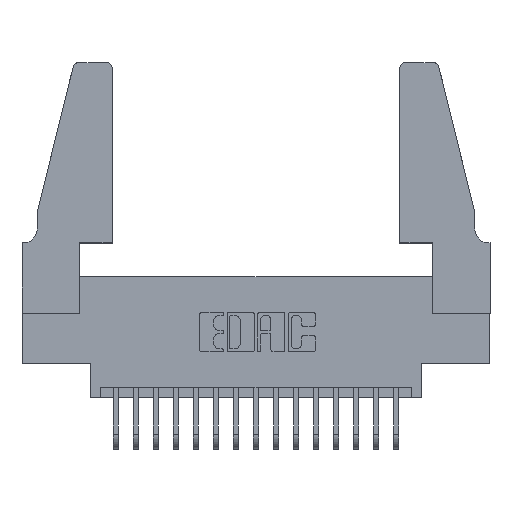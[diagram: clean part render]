
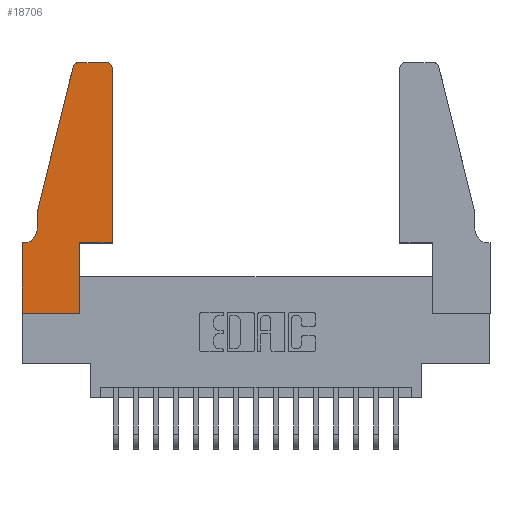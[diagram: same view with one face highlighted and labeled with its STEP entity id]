
A CAD part, top view. The second image highlights one B-rep face of the part: STEP entity #18706.
In plain terms, the highlighted planar face has unit normal (0, 0, 1).
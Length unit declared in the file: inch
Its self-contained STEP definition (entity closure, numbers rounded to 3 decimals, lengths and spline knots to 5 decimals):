
#60 = DIRECTION ( 'NONE',  ( -0.239, -0.971, 0. ) ) ;
#128 = CARTESIAN_POINT ( 'NONE',  ( 0.4505, 0.35, 0.37 ) ) ;
#160 = EDGE_CURVE ( 'NONE', #6069, #14616, #15178, .T. ) ;
#247 = EDGE_CURVE ( 'NONE', #14616, #1407, #3761, .T. ) ;
#434 = CIRCLE ( 'NONE', #5238, 0.03 ) ;
#468 = VECTOR ( 'NONE', #3571, 39.37008 ) ;
#499 = CARTESIAN_POINT ( 'NONE',  ( 0.0055, 0.42, 0.37 ) ) ;
#738 = CIRCLE ( 'NONE', #7041, 0.07 ) ;
#1019 = DIRECTION ( 'NONE',  ( 0., 0., 1. ) ) ;
#1141 = DIRECTION ( 'NONE',  ( -1., 0., 0. ) ) ;
#1270 = VERTEX_POINT ( 'NONE', #17193 ) ;
#1292 = VECTOR ( 'NONE', #11896, 39.37008 ) ;
#1400 = FACE_OUTER_BOUND ( 'NONE', #6857, .T. ) ;
#1407 = VERTEX_POINT ( 'NONE', #5744 ) ;
#1433 = CARTESIAN_POINT ( 'NONE',  ( 0.4505, 0.35, 0.37 ) ) ;
#1527 = EDGE_CURVE ( 'NONE', #12552, #3239, #3700, .T. ) ;
#1777 = VECTOR ( 'NONE', #12520, 39.37008 ) ;
#1873 = VECTOR ( 'NONE', #1141, 39.37008 ) ;
#2265 = VERTEX_POINT ( 'NONE', #14959 ) ;
#2568 = PLANE ( 'NONE',  #15104 ) ;
#2570 = VERTEX_POINT ( 'NONE', #6822 ) ;
#2880 = ORIENTED_EDGE ( 'NONE', *, *, #13255, .T. ) ;
#3009 = ORIENTED_EDGE ( 'NONE', *, *, #9297, .T. ) ;
#3200 = DIRECTION ( 'NONE',  ( 0., -1., 0. ) ) ;
#3239 = VERTEX_POINT ( 'NONE', #16061 ) ;
#3508 = CARTESIAN_POINT ( 'NONE',  ( 0.0755, 0.35, 0.37 ) ) ;
#3571 = DIRECTION ( 'NONE',  ( 1., 0., 0. ) ) ;
#3700 = LINE ( 'NONE', #17986, #8347 ) ;
#3761 = LINE ( 'NONE', #16652, #14265 ) ;
#3788 = ORIENTED_EDGE ( 'NONE', *, *, #7054, .T. ) ;
#4118 = DIRECTION ( 'NONE',  ( 0., 0., 1. ) ) ;
#4367 = LINE ( 'NONE', #3508, #1777 ) ;
#5176 = VECTOR ( 'NONE', #14884, 39.37008 ) ;
#5238 = AXIS2_PLACEMENT_3D ( 'NONE', #15968, #1019, #5418 ) ;
#5287 = LINE ( 'NONE', #1433, #1292 ) ;
#5418 = DIRECTION ( 'NONE',  ( 1., 0., 0. ) ) ;
#5697 = DIRECTION ( 'NONE',  ( 1., 0., 0. ) ) ;
#5744 = CARTESIAN_POINT ( 'NONE',  ( 0.2865, 0.35, 0.37 ) ) ;
#5806 = ORIENTED_EDGE ( 'NONE', *, *, #18556, .T. ) ;
#6069 = VERTEX_POINT ( 'NONE', #8183 ) ;
#6198 = ORIENTED_EDGE ( 'NONE', *, *, #1527, .T. ) ;
#6437 = ORIENTED_EDGE ( 'NONE', *, *, #14283, .T. ) ;
#6822 = CARTESIAN_POINT ( 'NONE',  ( 0.0755, 0.42, 0.37 ) ) ;
#6857 = EDGE_LOOP ( 'NONE', ( #16864, #3788, #6198, #16305, #12976, #6437, #3009, #13708, #15267, #5806, #18060, #2880 ) ) ;
#6881 = CARTESIAN_POINT ( 'NONE',  ( 0.25487, 1.22718, 0.37 ) ) ;
#7041 = AXIS2_PLACEMENT_3D ( 'NONE', #499, #16013, #14645 ) ;
#7054 = EDGE_CURVE ( 'NONE', #1270, #12552, #434, .T. ) ;
#7092 = DIRECTION ( 'NONE',  ( 0., 0., 1. ) ) ;
#7910 = VERTEX_POINT ( 'NONE', #15102 ) ;
#8183 = CARTESIAN_POINT ( 'NONE',  ( 0., 0., 0.37 ) ) ;
#8347 = VECTOR ( 'NONE', #60, 39.37008 ) ;
#8463 = EDGE_CURVE ( 'NONE', #3239, #2570, #17456, .T. ) ;
#8550 = LINE ( 'NONE', #18088, #10180 ) ;
#8596 = CARTESIAN_POINT ( 'NONE',  ( 0.0055, 0.35, 0.37 ) ) ;
#8775 = VERTEX_POINT ( 'NONE', #8596 ) ;
#9185 = EDGE_CURVE ( 'NONE', #17569, #19368, #5287, .T. ) ;
#9218 = DIRECTION ( 'NONE',  ( 0., 1., 0. ) ) ;
#9297 = EDGE_CURVE ( 'NONE', #7910, #6069, #8550, .T. ) ;
#10180 = VECTOR ( 'NONE', #3200, 39.37008 ) ;
#10377 = CARTESIAN_POINT ( 'NONE',  ( 0.4205, 1.22, 0.37 ) ) ;
#10914 = VECTOR ( 'NONE', #16899, 39.37008 ) ;
#10998 = EDGE_CURVE ( 'NONE', #2570, #8775, #738, .T. ) ;
#11688 = LINE ( 'NONE', #16017, #1873 ) ;
#11896 = DIRECTION ( 'NONE',  ( 0., 1., 0. ) ) ;
#12171 = LINE ( 'NONE', #14202, #468 ) ;
#12361 = EDGE_CURVE ( 'NONE', #2265, #1270, #11688, .T. ) ;
#12520 = DIRECTION ( 'NONE',  ( -1., 0., 0. ) ) ;
#12552 = VERTEX_POINT ( 'NONE', #6881 ) ;
#12976 = ORIENTED_EDGE ( 'NONE', *, *, #10998, .T. ) ;
#13255 = EDGE_CURVE ( 'NONE', #19368, #2265, #16784, .T. ) ;
#13708 = ORIENTED_EDGE ( 'NONE', *, *, #160, .T. ) ;
#14070 = AXIS2_PLACEMENT_3D ( 'NONE', #10377, #4118, #5697 ) ;
#14202 = CARTESIAN_POINT ( 'NONE',  ( 0.4505, 0.35, 0.37 ) ) ;
#14265 = VECTOR ( 'NONE', #9218, 39.37008 ) ;
#14268 = DIRECTION ( 'NONE',  ( 1., 0., 0. ) ) ;
#14283 = EDGE_CURVE ( 'NONE', #8775, #7910, #4367, .T. ) ;
#14616 = VERTEX_POINT ( 'NONE', #17322 ) ;
#14645 = DIRECTION ( 'NONE',  ( -1., 0., 0. ) ) ;
#14823 = CARTESIAN_POINT ( 'NONE',  ( 0., 0., 0.37 ) ) ;
#14884 = DIRECTION ( 'NONE',  ( 1., 0., 0. ) ) ;
#14959 = CARTESIAN_POINT ( 'NONE',  ( 0.4205, 1.25, 0.37 ) ) ;
#15102 = CARTESIAN_POINT ( 'NONE',  ( 0., 0.35, 0.37 ) ) ;
#15104 = AXIS2_PLACEMENT_3D ( 'NONE', #17271, #7092, #14268 ) ;
#15178 = LINE ( 'NONE', #14823, #5176 ) ;
#15267 = ORIENTED_EDGE ( 'NONE', *, *, #247, .T. ) ;
#15968 = CARTESIAN_POINT ( 'NONE',  ( 0.284, 1.22, 0.37 ) ) ;
#16013 = DIRECTION ( 'NONE',  ( 0., 0., -1. ) ) ;
#16017 = CARTESIAN_POINT ( 'NONE',  ( 0.2605, 1.25, 0.37 ) ) ;
#16061 = CARTESIAN_POINT ( 'NONE',  ( 0.0755, 0.5, 0.37 ) ) ;
#16305 = ORIENTED_EDGE ( 'NONE', *, *, #8463, .T. ) ;
#16652 = CARTESIAN_POINT ( 'NONE',  ( 0.2865, 0.35, 0.37 ) ) ;
#16784 = CIRCLE ( 'NONE', #14070, 0.03 ) ;
#16864 = ORIENTED_EDGE ( 'NONE', *, *, #12361, .T. ) ;
#16899 = DIRECTION ( 'NONE',  ( 0., -1., 0. ) ) ;
#17193 = CARTESIAN_POINT ( 'NONE',  ( 0.284, 1.25, 0.37 ) ) ;
#17271 = CARTESIAN_POINT ( 'NONE',  ( 0., 0.35, 0.37 ) ) ;
#17322 = CARTESIAN_POINT ( 'NONE',  ( 0.2865, 0., 0.37 ) ) ;
#17382 = CARTESIAN_POINT ( 'NONE',  ( 0.4505, 1.22, 0.37 ) ) ;
#17456 = LINE ( 'NONE', #18201, #10914 ) ;
#17569 = VERTEX_POINT ( 'NONE', #128 ) ;
#17986 = CARTESIAN_POINT ( 'NONE',  ( 0.0755, 0.5, 0.37 ) ) ;
#18060 = ORIENTED_EDGE ( 'NONE', *, *, #9185, .T. ) ;
#18088 = CARTESIAN_POINT ( 'NONE',  ( 0., 0., 0.37 ) ) ;
#18201 = CARTESIAN_POINT ( 'NONE',  ( 0.0755, 0.5, 0.37 ) ) ;
#18556 = EDGE_CURVE ( 'NONE', #1407, #17569, #12171, .T. ) ;
#18706 = ADVANCED_FACE ( 'NONE', ( #1400 ), #2568, .T. ) ;
#19368 = VERTEX_POINT ( 'NONE', #17382 ) ;
